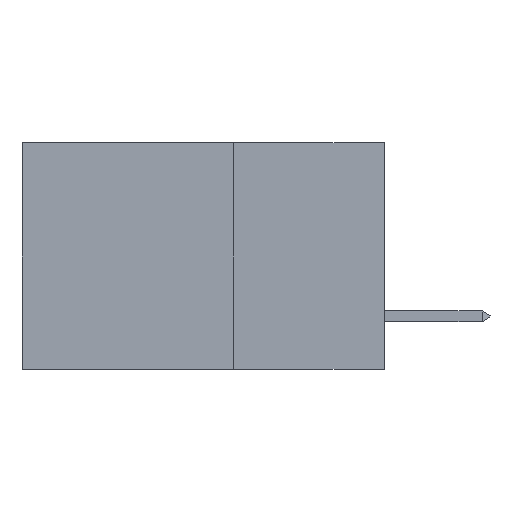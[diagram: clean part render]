
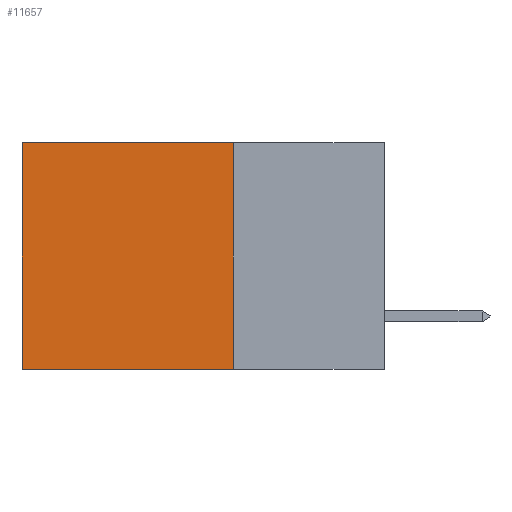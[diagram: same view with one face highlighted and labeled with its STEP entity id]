
A CAD part, left-side view. The second image highlights one B-rep face of the part: STEP entity #11657.
In plain terms, the highlighted planar face has unit normal (-1, 0, 0).
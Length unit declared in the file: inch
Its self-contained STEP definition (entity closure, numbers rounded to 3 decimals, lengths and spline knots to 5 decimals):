
#325 = EDGE_CURVE ( 'NONE', #15050, #14554, #7183, .T. ) ;
#375 = EDGE_LOOP ( 'NONE', ( #12360, #716, #2336, #12132 ) ) ;
#716 = ORIENTED_EDGE ( 'NONE', *, *, #2045, .F. ) ;
#914 = VECTOR ( 'NONE', #2431, 39.37008 ) ;
#989 = CARTESIAN_POINT ( 'NONE',  ( 0.2875, 0.25, -0.375 ) ) ;
#1240 = CARTESIAN_POINT ( 'NONE',  ( 0.2875, 0.6, -0.375 ) ) ;
#1348 = CARTESIAN_POINT ( 'NONE',  ( 0.2875, 0.25, -0.375 ) ) ;
#1383 = DIRECTION ( 'NONE',  ( 0., 0., -1. ) ) ;
#1660 = VERTEX_POINT ( 'NONE', #3582 ) ;
#2045 = EDGE_CURVE ( 'NONE', #14554, #1660, #11356, .T. ) ;
#2336 = ORIENTED_EDGE ( 'NONE', *, *, #325, .F. ) ;
#2431 = DIRECTION ( 'NONE',  ( 0., 0., -1. ) ) ;
#2833 = CARTESIAN_POINT ( 'NONE',  ( 0.2875, 0.25, 0. ) ) ;
#3470 = CARTESIAN_POINT ( 'NONE',  ( 0.2875, 0.25, 0. ) ) ;
#3500 = LINE ( 'NONE', #1240, #914 ) ;
#3582 = CARTESIAN_POINT ( 'NONE',  ( 0.2875, 0.6, -0.375 ) ) ;
#4047 = VECTOR ( 'NONE', #1383, 39.37008 ) ;
#4253 = AXIS2_PLACEMENT_3D ( 'NONE', #6023, #6121, #10618 ) ;
#6023 = CARTESIAN_POINT ( 'NONE',  ( 0.2875, 0.25, -0.375 ) ) ;
#6073 = FACE_OUTER_BOUND ( 'NONE', #375, .T. ) ;
#6121 = DIRECTION ( 'NONE',  ( 1., 0., 0. ) ) ;
#6374 = DIRECTION ( 'NONE',  ( 0., 1., 0. ) ) ;
#7183 = LINE ( 'NONE', #989, #4047 ) ;
#8234 = VECTOR ( 'NONE', #8666, 39.37008 ) ;
#8666 = DIRECTION ( 'NONE',  ( 0., 1., 0. ) ) ;
#9163 = VECTOR ( 'NONE', #6374, 39.37008 ) ;
#9642 = PLANE ( 'NONE',  #4253 ) ;
#10618 = DIRECTION ( 'NONE',  ( 0., 0., -1. ) ) ;
#11356 = LINE ( 'NONE', #12155, #8234 ) ;
#11657 = ADVANCED_FACE ( 'NONE', ( #6073 ), #9642, .F. ) ;
#12132 = ORIENTED_EDGE ( 'NONE', *, *, #12195, .T. ) ;
#12155 = CARTESIAN_POINT ( 'NONE',  ( 0.2875, 0.25, -0.375 ) ) ;
#12195 = EDGE_CURVE ( 'NONE', #15050, #14259, #14267, .T. ) ;
#12360 = ORIENTED_EDGE ( 'NONE', *, *, #14857, .T. ) ;
#13950 = CARTESIAN_POINT ( 'NONE',  ( 0.2875, 0.6, 0. ) ) ;
#14259 = VERTEX_POINT ( 'NONE', #13950 ) ;
#14267 = LINE ( 'NONE', #2833, #9163 ) ;
#14554 = VERTEX_POINT ( 'NONE', #1348 ) ;
#14857 = EDGE_CURVE ( 'NONE', #14259, #1660, #3500, .T. ) ;
#15050 = VERTEX_POINT ( 'NONE', #3470 ) ;
